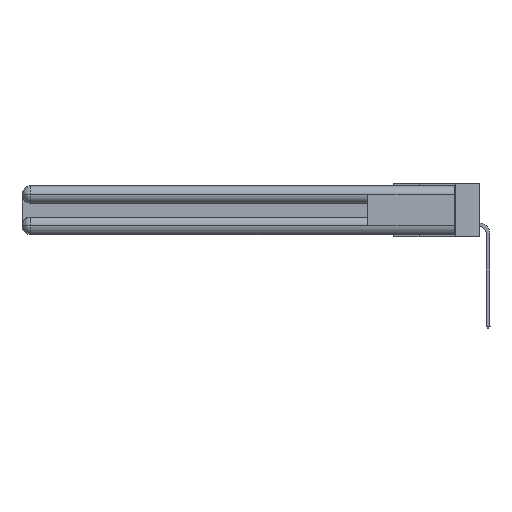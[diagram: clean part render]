
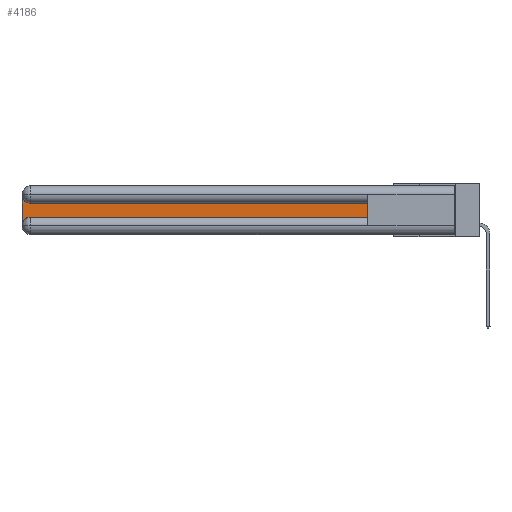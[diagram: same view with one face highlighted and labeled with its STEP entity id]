
A CAD part, left-side view. The second image highlights one B-rep face of the part: STEP entity #4186.
In plain terms, the highlighted planar face has unit normal (-1, 0, 0).
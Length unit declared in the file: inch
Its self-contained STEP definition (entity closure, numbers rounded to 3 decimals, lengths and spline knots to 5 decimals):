
#155 = CARTESIAN_POINT ( 'NONE',  ( 0.075, 3., -0.2175 ) ) ;
#311 = AXIS2_PLACEMENT_3D ( 'NONE', #13760, #8325, #13320 ) ;
#1388 = VECTOR ( 'NONE', #30873, 39.37008 ) ;
#1460 = CARTESIAN_POINT ( 'NONE',  ( 0.075, 0.6, -0.2175 ) ) ;
#2167 = LINE ( 'NONE', #1460, #21694 ) ;
#2805 = CARTESIAN_POINT ( 'NONE',  ( 0.075, 0.6, -0.2175 ) ) ;
#3744 = EDGE_CURVE ( 'NONE', #25510, #13941, #13768, .T. ) ;
#4186 = ADVANCED_FACE ( 'NONE', ( #18776 ), #13056, .F. ) ;
#4250 = CARTESIAN_POINT ( 'NONE',  ( 0.075, 2.94, -0.2175 ) ) ;
#4467 = CARTESIAN_POINT ( 'NONE',  ( 0.075, 0.6, -0.1225 ) ) ;
#5258 = AXIS2_PLACEMENT_3D ( 'NONE', #8323, #30976, #8100 ) ;
#5418 = DIRECTION ( 'NONE',  ( 0., -1., 0. ) ) ;
#5651 = CARTESIAN_POINT ( 'NONE',  ( 0.075, 3., -0.1225 ) ) ;
#6772 = LINE ( 'NONE', #2805, #9895 ) ;
#6796 = VERTEX_POINT ( 'NONE', #7376 ) ;
#7376 = CARTESIAN_POINT ( 'NONE',  ( 0.075, 2.94, -0.1225 ) ) ;
#8100 = DIRECTION ( 'NONE',  ( 0., 0., -1. ) ) ;
#8174 = DIRECTION ( 'NONE',  ( 0., 0., -1. ) ) ;
#8323 = CARTESIAN_POINT ( 'NONE',  ( 0.075, 2.94, -0.2775 ) ) ;
#8325 = DIRECTION ( 'NONE',  ( 1., 0., 0. ) ) ;
#9757 = VERTEX_POINT ( 'NONE', #29307 ) ;
#9895 = VECTOR ( 'NONE', #5418, 39.37008 ) ;
#10382 = CARTESIAN_POINT ( 'NONE',  ( 0.075, 0.6, -0.2175 ) ) ;
#13056 = PLANE ( 'NONE',  #26365 ) ;
#13320 = DIRECTION ( 'NONE',  ( 0., 0., -1. ) ) ;
#13760 = CARTESIAN_POINT ( 'NONE',  ( 0.075, 2.94, -0.0625 ) ) ;
#13768 = CIRCLE ( 'NONE', #5258, 0.06 ) ;
#13941 = VERTEX_POINT ( 'NONE', #4250 ) ;
#14448 = EDGE_LOOP ( 'NONE', ( #32087, #28085, #21364, #25584, #16480, #18255 ) ) ;
#14830 = EDGE_CURVE ( 'NONE', #9757, #6796, #21607, .T. ) ;
#14967 = EDGE_CURVE ( 'NONE', #13941, #15660, #6772, .T. ) ;
#15660 = VERTEX_POINT ( 'NONE', #10382 ) ;
#15793 = EDGE_CURVE ( 'NONE', #6796, #23348, #25409, .T. ) ;
#16480 = ORIENTED_EDGE ( 'NONE', *, *, #14967, .T. ) ;
#18255 = ORIENTED_EDGE ( 'NONE', *, *, #23362, .T. ) ;
#18776 = FACE_OUTER_BOUND ( 'NONE', #14448, .T. ) ;
#19795 = CARTESIAN_POINT ( 'NONE',  ( 0.075, 3., -0.2775 ) ) ;
#21364 = ORIENTED_EDGE ( 'NONE', *, *, #24615, .T. ) ;
#21607 = LINE ( 'NONE', #4467, #30556 ) ;
#21694 = VECTOR ( 'NONE', #26616, 39.37008 ) ;
#23348 = VERTEX_POINT ( 'NONE', #28474 ) ;
#23362 = EDGE_CURVE ( 'NONE', #15660, #9757, #2167, .T. ) ;
#24615 = EDGE_CURVE ( 'NONE', #23348, #25510, #27097, .T. ) ;
#25409 = CIRCLE ( 'NONE', #311, 0.06 ) ;
#25510 = VERTEX_POINT ( 'NONE', #19795 ) ;
#25584 = ORIENTED_EDGE ( 'NONE', *, *, #3744, .T. ) ;
#26365 = AXIS2_PLACEMENT_3D ( 'NONE', #5651, #30599, #8174 ) ;
#26616 = DIRECTION ( 'NONE',  ( 0., 0., 1. ) ) ;
#27097 = LINE ( 'NONE', #155, #1388 ) ;
#28085 = ORIENTED_EDGE ( 'NONE', *, *, #15793, .T. ) ;
#28474 = CARTESIAN_POINT ( 'NONE',  ( 0.075, 3., -0.0625 ) ) ;
#29307 = CARTESIAN_POINT ( 'NONE',  ( 0.075, 0.6, -0.1225 ) ) ;
#30556 = VECTOR ( 'NONE', #31707, 39.37008 ) ;
#30599 = DIRECTION ( 'NONE',  ( 1., 0., 0. ) ) ;
#30873 = DIRECTION ( 'NONE',  ( 0., 0., -1. ) ) ;
#30976 = DIRECTION ( 'NONE',  ( 1., 0., 0. ) ) ;
#31707 = DIRECTION ( 'NONE',  ( 0., 1., 0. ) ) ;
#32087 = ORIENTED_EDGE ( 'NONE', *, *, #14830, .T. ) ;
